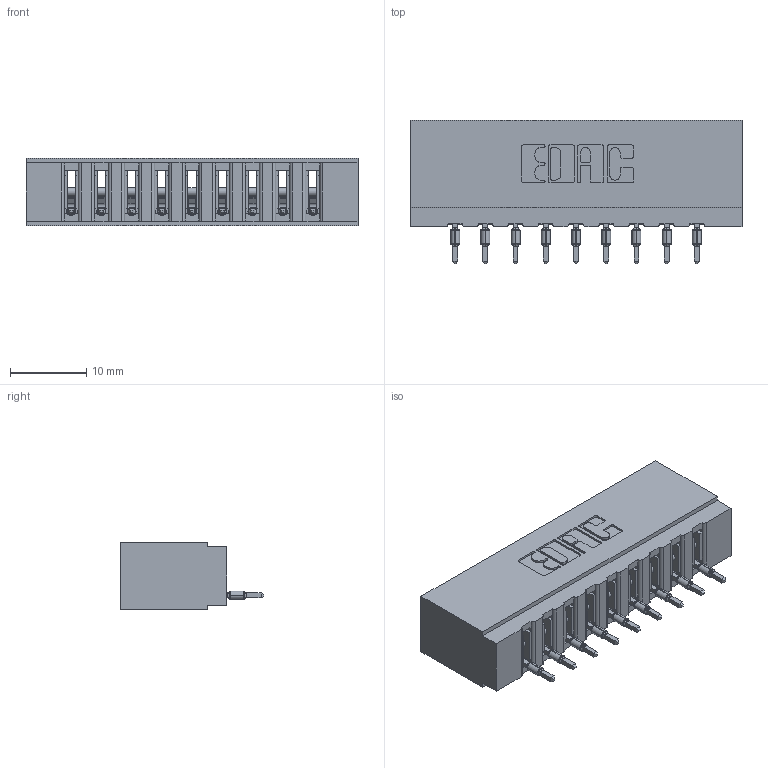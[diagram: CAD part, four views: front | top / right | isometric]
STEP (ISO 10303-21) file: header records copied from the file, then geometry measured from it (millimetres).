
FILE_DESCRIPTION (( 'STEP AP203' ), '1' );
FILE_NAME ('717-009-560-106.STEP', '2020-03-13T17:52:51', ( '' ), ( '' ), 'SwSTEP 2.0', 'SolidWorks 2016', '' );
FILE_SCHEMA (( 'CONFIG_CONTROL_DESIGN' ));
Length unit declared in the file: inch
Products named in the file (3): 745-292-001_560; 717-009-560-106; 717 Part_Insulator Option - 06
Assembly tree (10 placements, depth 2):
  717-009-560-106
    717 Part_Insulator Option - 06
    745-292-001_560  x9
Bounding box: 43.54 x 18.78 x 8.89 mm (x, y, z)
Volume: 3853.9 mm3; surface area: 5200.4 mm2
Topology: 10 solids, 10 shells, 1192 faces, 3311 edges, 2110 vertices
Faces by surface type: plane 711, cylinder 247, bspline 180, torus 54
Entity records: 19926 total; most frequent: CARTESIAN_POINT 4012, ORIENTED_EDGE 3390, DIRECTION 2977, EDGE_CURVE 1695, LINE 1451, VECTOR 1451, VERTEX_POINT 1086, AXIS2_PLACEMENT_3D 763
